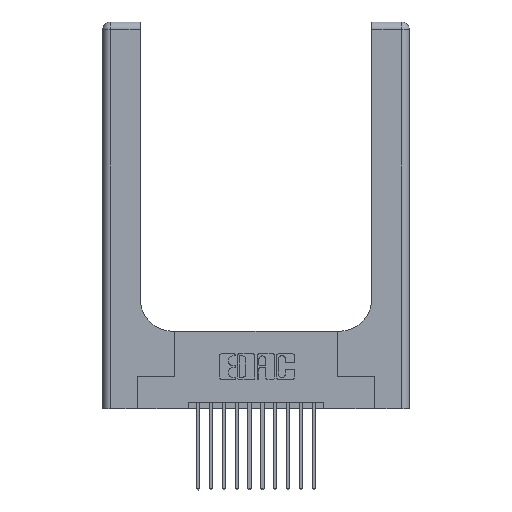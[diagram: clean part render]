
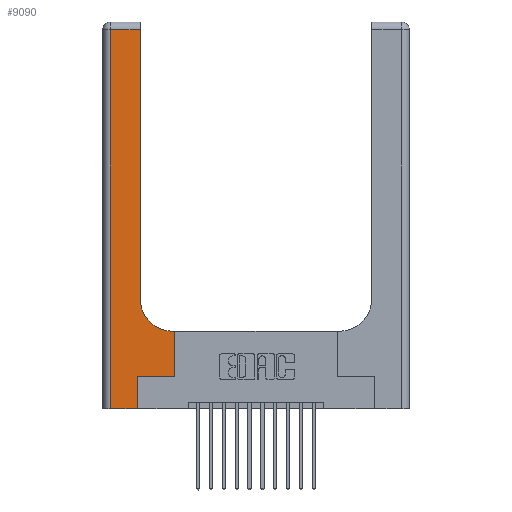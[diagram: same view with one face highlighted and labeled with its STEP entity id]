
A CAD part, top view. The second image highlights one B-rep face of the part: STEP entity #9090.
In plain terms, the highlighted planar face has unit normal (0, 0, 1).
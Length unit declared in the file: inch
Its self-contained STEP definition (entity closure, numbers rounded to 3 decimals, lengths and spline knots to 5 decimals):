
#88 = VERTEX_POINT ( 'NONE', #6809 ) ;
#179 = LINE ( 'NONE', #12471, #11339 ) ;
#245 = DIRECTION ( 'NONE',  ( 0., -1., 0. ) ) ;
#253 = VECTOR ( 'NONE', #11142, 39.37008 ) ;
#370 = CARTESIAN_POINT ( 'NONE',  ( 0., 2.94, 0.37 ) ) ;
#602 = ORIENTED_EDGE ( 'NONE', *, *, #2919, .T. ) ;
#701 = ORIENTED_EDGE ( 'NONE', *, *, #4012, .T. ) ;
#1487 = DIRECTION ( 'NONE',  ( -1., 0., 0. ) ) ;
#1610 = PLANE ( 'NONE',  #5921 ) ;
#1643 = CARTESIAN_POINT ( 'NONE',  ( 0.2915, 0.85, 0.37 ) ) ;
#1838 = CARTESIAN_POINT ( 'NONE',  ( 0.2915, 2.94, 0.37 ) ) ;
#2649 = VERTEX_POINT ( 'NONE', #14069 ) ;
#2729 = EDGE_CURVE ( 'NONE', #12615, #7468, #4525, .T. ) ;
#2919 = EDGE_CURVE ( 'NONE', #3408, #6322, #6183, .T. ) ;
#3239 = DIRECTION ( 'NONE',  ( 0., 1., 0. ) ) ;
#3408 = VERTEX_POINT ( 'NONE', #14105 ) ;
#3508 = LINE ( 'NONE', #6397, #9393 ) ;
#4012 = EDGE_CURVE ( 'NONE', #88, #8635, #16212, .T. ) ;
#4154 = CARTESIAN_POINT ( 'NONE',  ( 0., 3., 0.37 ) ) ;
#4233 = ORIENTED_EDGE ( 'NONE', *, *, #7511, .T. ) ;
#4374 = VECTOR ( 'NONE', #10741, 39.37008 ) ;
#4409 = ORIENTED_EDGE ( 'NONE', *, *, #4856, .T. ) ;
#4525 = CIRCLE ( 'NONE', #10146, 0.25 ) ;
#4856 = EDGE_CURVE ( 'NONE', #7468, #8849, #11002, .T. ) ;
#4954 = EDGE_CURVE ( 'NONE', #8849, #3408, #13741, .T. ) ;
#5276 = CARTESIAN_POINT ( 'NONE',  ( 0., 0., 0.37 ) ) ;
#5701 = CARTESIAN_POINT ( 'NONE',  ( 0.06, 3., 0.37 ) ) ;
#5921 = AXIS2_PLACEMENT_3D ( 'NONE', #4154, #6785, #1487 ) ;
#6183 = LINE ( 'NONE', #5701, #8343 ) ;
#6225 = DIRECTION ( 'NONE',  ( 1., 0., 0. ) ) ;
#6322 = VERTEX_POINT ( 'NONE', #15119 ) ;
#6397 = CARTESIAN_POINT ( 'NONE',  ( 0.2915, 0.6, 0.37 ) ) ;
#6424 = ORIENTED_EDGE ( 'NONE', *, *, #2729, .T. ) ;
#6655 = LINE ( 'NONE', #9383, #4374 ) ;
#6717 = DIRECTION ( 'NONE',  ( 1., 0., 0. ) ) ;
#6785 = DIRECTION ( 'NONE',  ( 0., 0., -1. ) ) ;
#6809 = CARTESIAN_POINT ( 'NONE',  ( 0.269, 0.25, 0.37 ) ) ;
#7094 = DIRECTION ( 'NONE',  ( 1., 0., 0. ) ) ;
#7468 = VERTEX_POINT ( 'NONE', #1643 ) ;
#7511 = EDGE_CURVE ( 'NONE', #11560, #88, #179, .T. ) ;
#7619 = VECTOR ( 'NONE', #16302, 39.37008 ) ;
#8343 = VECTOR ( 'NONE', #245, 39.37008 ) ;
#8534 = EDGE_CURVE ( 'NONE', #2649, #12615, #3508, .T. ) ;
#8635 = VERTEX_POINT ( 'NONE', #9641 ) ;
#8849 = VERTEX_POINT ( 'NONE', #1838 ) ;
#9090 = ADVANCED_FACE ( 'NONE', ( #11537 ), #1610, .F. ) ;
#9383 = CARTESIAN_POINT ( 'NONE',  ( 0.5585, 0.25, 0.37 ) ) ;
#9393 = VECTOR ( 'NONE', #10467, 39.37008 ) ;
#9641 = CARTESIAN_POINT ( 'NONE',  ( 0.5585, 0.25, 0.37 ) ) ;
#10146 = AXIS2_PLACEMENT_3D ( 'NONE', #12975, #16936, #6225 ) ;
#10375 = EDGE_CURVE ( 'NONE', #8635, #2649, #6655, .T. ) ;
#10467 = DIRECTION ( 'NONE',  ( -1., 0., 0. ) ) ;
#10739 = VECTOR ( 'NONE', #6717, 39.37008 ) ;
#10741 = DIRECTION ( 'NONE',  ( 0., 1., 0. ) ) ;
#11002 = LINE ( 'NONE', #16360, #253 ) ;
#11005 = CARTESIAN_POINT ( 'NONE',  ( 0.269, 0., 0.37 ) ) ;
#11029 = CARTESIAN_POINT ( 'NONE',  ( 0.269, 0.25, 0.37 ) ) ;
#11142 = DIRECTION ( 'NONE',  ( 0., 1., 0. ) ) ;
#11339 = VECTOR ( 'NONE', #3239, 39.37008 ) ;
#11537 = FACE_OUTER_BOUND ( 'NONE', #16505, .T. ) ;
#11560 = VERTEX_POINT ( 'NONE', #11005 ) ;
#12471 = CARTESIAN_POINT ( 'NONE',  ( 0.269, 0., 0.37 ) ) ;
#12615 = VERTEX_POINT ( 'NONE', #16256 ) ;
#12741 = VECTOR ( 'NONE', #7094, 39.37008 ) ;
#12975 = CARTESIAN_POINT ( 'NONE',  ( 0.5415, 0.85, 0.37 ) ) ;
#12981 = ORIENTED_EDGE ( 'NONE', *, *, #4954, .T. ) ;
#13741 = LINE ( 'NONE', #370, #7619 ) ;
#13916 = ORIENTED_EDGE ( 'NONE', *, *, #15627, .T. ) ;
#14069 = CARTESIAN_POINT ( 'NONE',  ( 0.5585, 0.6, 0.37 ) ) ;
#14105 = CARTESIAN_POINT ( 'NONE',  ( 0.06, 2.94, 0.37 ) ) ;
#14312 = LINE ( 'NONE', #5276, #10739 ) ;
#15119 = CARTESIAN_POINT ( 'NONE',  ( 0.06, 0., 0.37 ) ) ;
#15178 = ORIENTED_EDGE ( 'NONE', *, *, #10375, .T. ) ;
#15295 = ORIENTED_EDGE ( 'NONE', *, *, #8534, .T. ) ;
#15627 = EDGE_CURVE ( 'NONE', #6322, #11560, #14312, .T. ) ;
#16212 = LINE ( 'NONE', #11029, #12741 ) ;
#16256 = CARTESIAN_POINT ( 'NONE',  ( 0.5415, 0.6, 0.37 ) ) ;
#16302 = DIRECTION ( 'NONE',  ( -1., 0., 0. ) ) ;
#16360 = CARTESIAN_POINT ( 'NONE',  ( 0.2915, 3., 0.37 ) ) ;
#16505 = EDGE_LOOP ( 'NONE', ( #4409, #12981, #602, #13916, #4233, #701, #15178, #15295, #6424 ) ) ;
#16936 = DIRECTION ( 'NONE',  ( 0., 0., -1. ) ) ;
